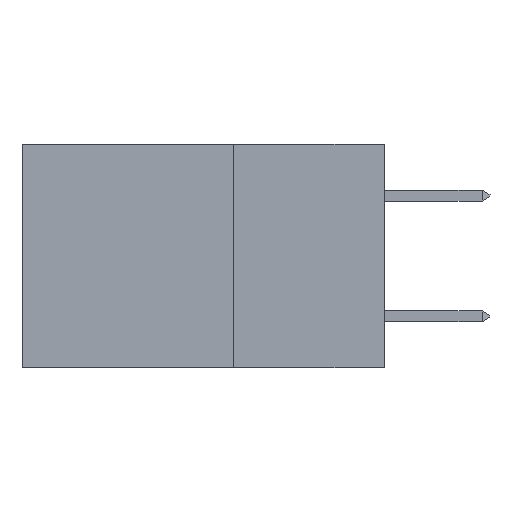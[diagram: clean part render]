
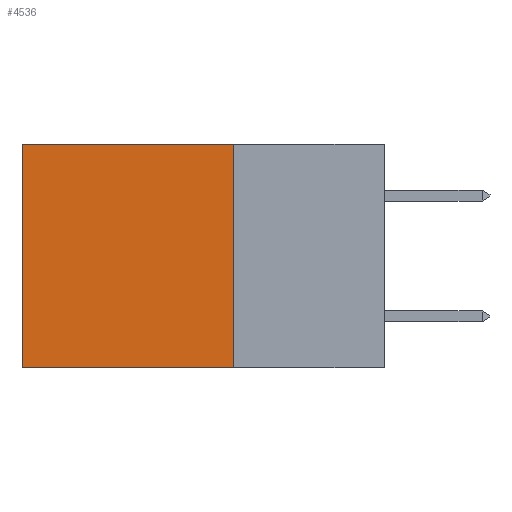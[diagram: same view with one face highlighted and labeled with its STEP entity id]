
A CAD part, left-side view. The second image highlights one B-rep face of the part: STEP entity #4536.
In plain terms, the highlighted planar face has unit normal (-1, 0, 0).
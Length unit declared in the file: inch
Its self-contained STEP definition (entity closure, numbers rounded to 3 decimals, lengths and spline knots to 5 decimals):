
#45 = CARTESIAN_POINT ( 'NONE',  ( 0.2875, 0.6, 0. ) ) ;
#61 = VERTEX_POINT ( 'NONE', #7105 ) ;
#459 = CARTESIAN_POINT ( 'NONE',  ( 0.2875, 0.6, -0.37 ) ) ;
#540 = VERTEX_POINT ( 'NONE', #459 ) ;
#718 = EDGE_CURVE ( 'NONE', #61, #540, #1544, .T. ) ;
#812 = VERTEX_POINT ( 'NONE', #6093 ) ;
#922 = ORIENTED_EDGE ( 'NONE', *, *, #7227, .T. ) ;
#1127 = FACE_OUTER_BOUND ( 'NONE', #10768, .T. ) ;
#1534 = LINE ( 'NONE', #2077, #6185 ) ;
#1544 = LINE ( 'NONE', #45, #5883 ) ;
#1585 = DIRECTION ( 'NONE',  ( 0., 0., -1. ) ) ;
#2077 = CARTESIAN_POINT ( 'NONE',  ( 0.2875, 0.25, 0. ) ) ;
#2103 = VERTEX_POINT ( 'NONE', #8899 ) ;
#3552 = DIRECTION ( 'NONE',  ( 0., 0., -1. ) ) ;
#3569 = DIRECTION ( 'NONE',  ( 1., 0., 0. ) ) ;
#3608 = PLANE ( 'NONE',  #4836 ) ;
#3637 = CARTESIAN_POINT ( 'NONE',  ( 0.2875, 0.25, 0. ) ) ;
#4536 = ADVANCED_FACE ( 'NONE', ( #1127 ), #3608, .F. ) ;
#4836 = AXIS2_PLACEMENT_3D ( 'NONE', #3637, #3569, #3552 ) ;
#5078 = DIRECTION ( 'NONE',  ( 0., 1., 0. ) ) ;
#5120 = VECTOR ( 'NONE', #5847, 39.37008 ) ;
#5847 = DIRECTION ( 'NONE',  ( 0., 1., 0. ) ) ;
#5883 = VECTOR ( 'NONE', #1585, 39.37008 ) ;
#6018 = CARTESIAN_POINT ( 'NONE',  ( 0.2875, 0.25, 0. ) ) ;
#6093 = CARTESIAN_POINT ( 'NONE',  ( 0.2875, 0.25, -0.37 ) ) ;
#6185 = VECTOR ( 'NONE', #11342, 39.37008 ) ;
#6962 = LINE ( 'NONE', #6018, #9093 ) ;
#7105 = CARTESIAN_POINT ( 'NONE',  ( 0.2875, 0.6, 0. ) ) ;
#7227 = EDGE_CURVE ( 'NONE', #2103, #61, #6962, .T. ) ;
#7279 = ORIENTED_EDGE ( 'NONE', *, *, #10987, .F. ) ;
#8613 = CARTESIAN_POINT ( 'NONE',  ( 0.2875, 0.25, -0.37 ) ) ;
#8899 = CARTESIAN_POINT ( 'NONE',  ( 0.2875, 0.25, 0. ) ) ;
#9067 = ORIENTED_EDGE ( 'NONE', *, *, #718, .T. ) ;
#9093 = VECTOR ( 'NONE', #5078, 39.37008 ) ;
#9972 = LINE ( 'NONE', #8613, #5120 ) ;
#10500 = EDGE_CURVE ( 'NONE', #812, #540, #9972, .T. ) ;
#10768 = EDGE_LOOP ( 'NONE', ( #9067, #10844, #7279, #922 ) ) ;
#10844 = ORIENTED_EDGE ( 'NONE', *, *, #10500, .F. ) ;
#10987 = EDGE_CURVE ( 'NONE', #2103, #812, #1534, .T. ) ;
#11342 = DIRECTION ( 'NONE',  ( 0., 0., -1. ) ) ;
